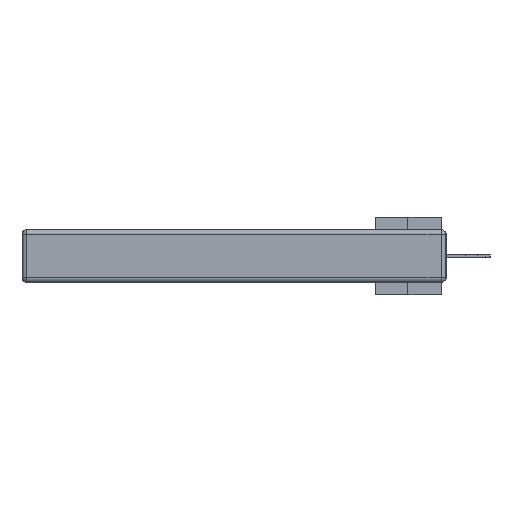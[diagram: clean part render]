
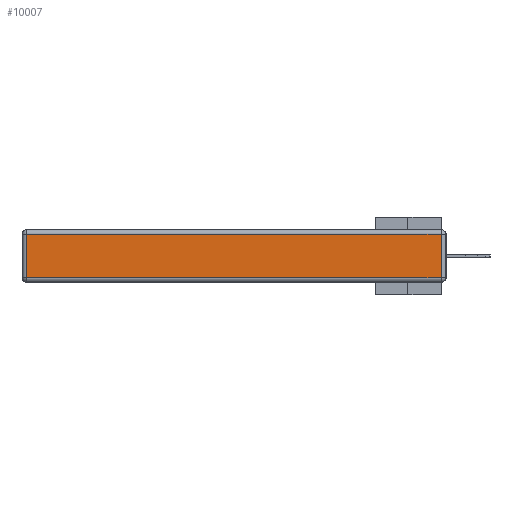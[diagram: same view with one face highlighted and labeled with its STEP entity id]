
A CAD part, left-side view. The second image highlights one B-rep face of the part: STEP entity #10007.
In plain terms, the highlighted planar face has unit normal (-1, 0, 0).
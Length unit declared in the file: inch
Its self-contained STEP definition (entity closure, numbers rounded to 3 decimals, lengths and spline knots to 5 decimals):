
#1538 = DIRECTION ( 'NONE',  ( 0., 0., 1. ) ) ;
#1563 = CARTESIAN_POINT ( 'NONE',  ( 0., 0.03, -0.03 ) ) ;
#2578 = CARTESIAN_POINT ( 'NONE',  ( 0., 2.72, -0.03 ) ) ;
#2663 = CARTESIAN_POINT ( 'NONE',  ( 0., 0.03, -0.343 ) ) ;
#3523 = VERTEX_POINT ( 'NONE', #18400 ) ;
#4189 = EDGE_CURVE ( 'NONE', #3523, #17009, #24479, .T. ) ;
#4422 = VERTEX_POINT ( 'NONE', #2578 ) ;
#4826 = VECTOR ( 'NONE', #32323, 39.37008 ) ;
#5319 = EDGE_CURVE ( 'NONE', #17009, #13579, #26842, .T. ) ;
#5599 = DIRECTION ( 'NONE',  ( 0., -1., 0. ) ) ;
#5746 = ORIENTED_EDGE ( 'NONE', *, *, #18492, .T. ) ;
#6774 = VECTOR ( 'NONE', #5599, 39.37008 ) ;
#7868 = DIRECTION ( 'NONE',  ( 0., 0., -1. ) ) ;
#8619 = DIRECTION ( 'NONE',  ( -1., 0., 0. ) ) ;
#9181 = EDGE_CURVE ( 'NONE', #4422, #3523, #18637, .T. ) ;
#10007 = ADVANCED_FACE ( 'NONE', ( #24176 ), #14081, .T. ) ;
#11178 = CARTESIAN_POINT ( 'NONE',  ( 0., 0.03, -0.313 ) ) ;
#13579 = VERTEX_POINT ( 'NONE', #1563 ) ;
#14081 = PLANE ( 'NONE',  #26084 ) ;
#17009 = VERTEX_POINT ( 'NONE', #11178 ) ;
#18400 = CARTESIAN_POINT ( 'NONE',  ( 0., 2.72, -0.313 ) ) ;
#18492 = EDGE_CURVE ( 'NONE', #13579, #4422, #23177, .T. ) ;
#18637 = LINE ( 'NONE', #29770, #29051 ) ;
#18707 = ORIENTED_EDGE ( 'NONE', *, *, #9181, .T. ) ;
#21986 = VECTOR ( 'NONE', #22996, 39.37008 ) ;
#22002 = CARTESIAN_POINT ( 'NONE',  ( 0., 0., -0.313 ) ) ;
#22082 = ORIENTED_EDGE ( 'NONE', *, *, #5319, .T. ) ;
#22658 = CARTESIAN_POINT ( 'NONE',  ( 0., 2.75, -0.03 ) ) ;
#22996 = DIRECTION ( 'NONE',  ( 0., 1., 0. ) ) ;
#23177 = LINE ( 'NONE', #22658, #21986 ) ;
#24128 = ORIENTED_EDGE ( 'NONE', *, *, #4189, .T. ) ;
#24176 = FACE_OUTER_BOUND ( 'NONE', #32800, .T. ) ;
#24479 = LINE ( 'NONE', #22002, #6774 ) ;
#24511 = CARTESIAN_POINT ( 'NONE',  ( 0., 0., -0.343 ) ) ;
#26084 = AXIS2_PLACEMENT_3D ( 'NONE', #24511, #8619, #1538 ) ;
#26842 = LINE ( 'NONE', #2663, #4826 ) ;
#29051 = VECTOR ( 'NONE', #7868, 39.37008 ) ;
#29770 = CARTESIAN_POINT ( 'NONE',  ( 0., 2.72, -0.343 ) ) ;
#32323 = DIRECTION ( 'NONE',  ( 0., 0., 1. ) ) ;
#32800 = EDGE_LOOP ( 'NONE', ( #24128, #22082, #5746, #18707 ) ) ;
